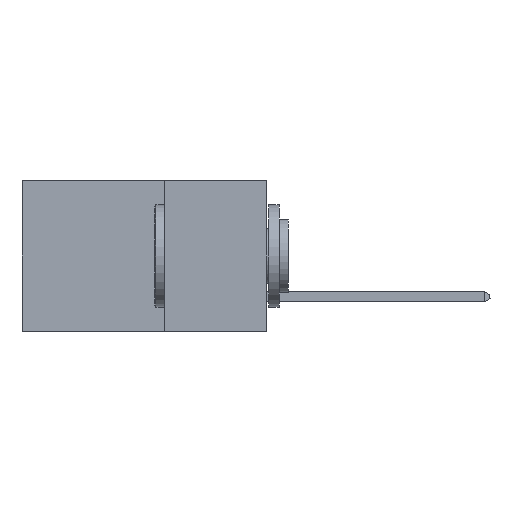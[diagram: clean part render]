
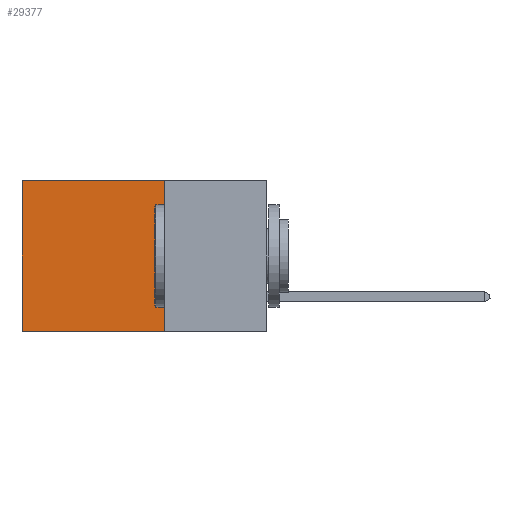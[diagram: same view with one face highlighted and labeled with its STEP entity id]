
A CAD part, left-side view. The second image highlights one B-rep face of the part: STEP entity #29377.
In plain terms, the highlighted planar face has unit normal (-1, 0, 0).
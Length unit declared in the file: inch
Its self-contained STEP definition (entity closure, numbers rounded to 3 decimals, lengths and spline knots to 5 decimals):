
#781 = VERTEX_POINT ( 'NONE', #32294 ) ;
#866 = DIRECTION ( 'NONE',  ( 0., 1., 0. ) ) ;
#1074 = VERTEX_POINT ( 'NONE', #25284 ) ;
#2279 = EDGE_CURVE ( 'NONE', #1074, #35878, #32416, .T. ) ;
#3449 = CARTESIAN_POINT ( 'NONE',  ( 0.2875, 0.6, 0. ) ) ;
#4770 = EDGE_CURVE ( 'NONE', #781, #10952, #17192, .T. ) ;
#9065 = DIRECTION ( 'NONE',  ( 0., 0., -1. ) ) ;
#9237 = VECTOR ( 'NONE', #26547, 39.37008 ) ;
#9629 = DIRECTION ( 'NONE',  ( 0., 0., -1. ) ) ;
#9965 = ORIENTED_EDGE ( 'NONE', *, *, #24971, .F. ) ;
#10526 = LINE ( 'NONE', #3449, #28233 ) ;
#10725 = LINE ( 'NONE', #27845, #33486 ) ;
#10952 = VERTEX_POINT ( 'NONE', #32802 ) ;
#11961 = PLANE ( 'NONE',  #16749 ) ;
#12181 = DIRECTION ( 'NONE',  ( 0., 0., -1. ) ) ;
#12356 = CARTESIAN_POINT ( 'NONE',  ( 0.2875, 0.6, 0. ) ) ;
#12692 = ORIENTED_EDGE ( 'NONE', *, *, #36537, .T. ) ;
#14124 = FACE_OUTER_BOUND ( 'NONE', #24240, .T. ) ;
#16749 = AXIS2_PLACEMENT_3D ( 'NONE', #32733, #36051, #9065 ) ;
#17192 = LINE ( 'NONE', #20294, #9237 ) ;
#20294 = CARTESIAN_POINT ( 'NONE',  ( 0.2875, 0.25, -0.37 ) ) ;
#23586 = VECTOR ( 'NONE', #866, 39.37008 ) ;
#24240 = EDGE_LOOP ( 'NONE', ( #12692, #30906, #9965, #28653 ) ) ;
#24539 = CARTESIAN_POINT ( 'NONE',  ( 0.2875, 0.25, 0. ) ) ;
#24971 = EDGE_CURVE ( 'NONE', #1074, #781, #10725, .T. ) ;
#25284 = CARTESIAN_POINT ( 'NONE',  ( 0.2875, 0.25, 0. ) ) ;
#26547 = DIRECTION ( 'NONE',  ( 0., 1., 0. ) ) ;
#27845 = CARTESIAN_POINT ( 'NONE',  ( 0.2875, 0.25, 0. ) ) ;
#28233 = VECTOR ( 'NONE', #12181, 39.37008 ) ;
#28653 = ORIENTED_EDGE ( 'NONE', *, *, #2279, .T. ) ;
#29377 = ADVANCED_FACE ( 'NONE', ( #14124 ), #11961, .F. ) ;
#30906 = ORIENTED_EDGE ( 'NONE', *, *, #4770, .F. ) ;
#32294 = CARTESIAN_POINT ( 'NONE',  ( 0.2875, 0.25, -0.37 ) ) ;
#32416 = LINE ( 'NONE', #24539, #23586 ) ;
#32733 = CARTESIAN_POINT ( 'NONE',  ( 0.2875, 0.25, 0. ) ) ;
#32802 = CARTESIAN_POINT ( 'NONE',  ( 0.2875, 0.6, -0.37 ) ) ;
#33486 = VECTOR ( 'NONE', #9629, 39.37008 ) ;
#35878 = VERTEX_POINT ( 'NONE', #12356 ) ;
#36051 = DIRECTION ( 'NONE',  ( 1., 0., 0. ) ) ;
#36537 = EDGE_CURVE ( 'NONE', #35878, #10952, #10526, .T. ) ;
